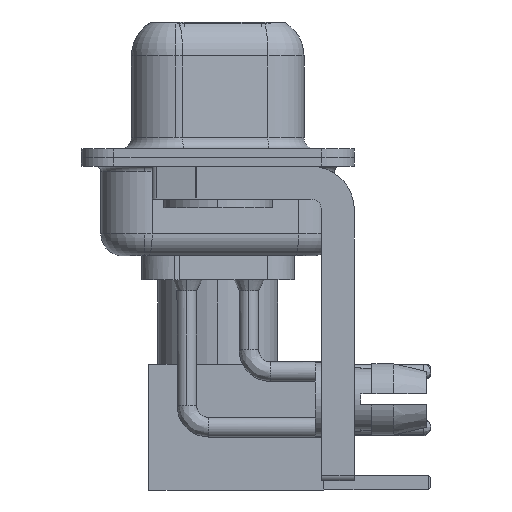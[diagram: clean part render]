
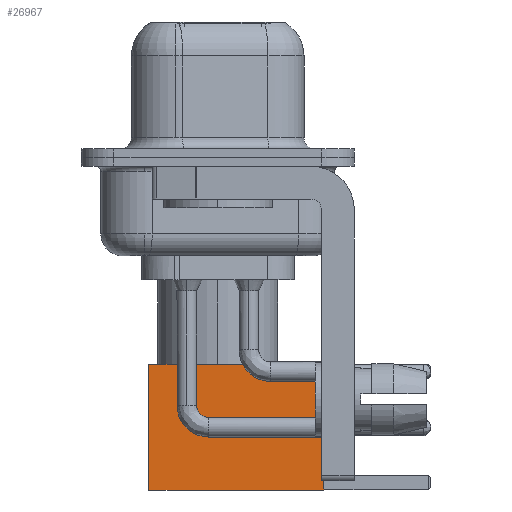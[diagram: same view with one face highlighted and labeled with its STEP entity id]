
A CAD part, left-side view. The second image highlights one B-rep face of the part: STEP entity #26967.
In plain terms, the highlighted face is planar.
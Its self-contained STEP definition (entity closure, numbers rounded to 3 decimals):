
#485 = CARTESIAN_POINT ( 'NONE',  ( 2.875, 2.875, 0. ) ) ;
#656 = VECTOR ( 'NONE', #3572, 1000. ) ;
#662 = LINE ( 'NONE', #13475, #1100 ) ;
#1100 = VECTOR ( 'NONE', #22975, 1000. ) ;
#1269 = CARTESIAN_POINT ( 'NONE',  ( -2.875, 2.875, 0. ) ) ;
#2920 = ORIENTED_EDGE ( 'NONE', *, *, #26882, .T. ) ;
#3572 = DIRECTION ( 'NONE',  ( 0., 0., -1. ) ) ;
#5492 = ORIENTED_EDGE ( 'NONE', *, *, #26355, .T. ) ;
#6103 = PLANE ( 'NONE',  #18853 ) ;
#7157 = VERTEX_POINT ( 'NONE', #485 ) ;
#7866 = CARTESIAN_POINT ( 'NONE',  ( 2.875, 2.875, 8. ) ) ;
#8279 = CARTESIAN_POINT ( 'NONE',  ( -2.875, 2.875, 0. ) ) ;
#9810 = LINE ( 'NONE', #1269, #19902 ) ;
#10529 = FACE_OUTER_BOUND ( 'NONE', #19339, .T. ) ;
#11374 = VERTEX_POINT ( 'NONE', #7866 ) ;
#12388 = DIRECTION ( 'NONE',  ( 0., 0., 1. ) ) ;
#12498 = ORIENTED_EDGE ( 'NONE', *, *, #13715, .F. ) ;
#12614 = VERTEX_POINT ( 'NONE', #14843 ) ;
#13475 = CARTESIAN_POINT ( 'NONE',  ( 0., 2.875, 0. ) ) ;
#13715 = EDGE_CURVE ( 'NONE', #12614, #16427, #9810, .T. ) ;
#14843 = CARTESIAN_POINT ( 'NONE',  ( -2.875, 2.875, 8. ) ) ;
#16333 = DIRECTION ( 'NONE',  ( -1., 0., 0. ) ) ;
#16427 = VERTEX_POINT ( 'NONE', #8279 ) ;
#16825 = CARTESIAN_POINT ( 'NONE',  ( 2.875, 2.875, 0. ) ) ;
#16898 = CARTESIAN_POINT ( 'NONE',  ( 0., 2.875, 8. ) ) ;
#18502 = DIRECTION ( 'NONE',  ( 0., 0., -1. ) ) ;
#18853 = AXIS2_PLACEMENT_3D ( 'NONE', #16825, #23356, #12388 ) ;
#19028 = LINE ( 'NONE', #16898, #24351 ) ;
#19339 = EDGE_LOOP ( 'NONE', ( #2920, #5492, #12498, #24939 ) ) ;
#19902 = VECTOR ( 'NONE', #18502, 1000. ) ;
#22975 = DIRECTION ( 'NONE',  ( -1., 0., 0. ) ) ;
#23356 = DIRECTION ( 'NONE',  ( 0., 1., 0. ) ) ;
#24351 = VECTOR ( 'NONE', #16333, 1000. ) ;
#24939 = ORIENTED_EDGE ( 'NONE', *, *, #27684, .F. ) ;
#25080 = LINE ( 'NONE', #25361, #656 ) ;
#25361 = CARTESIAN_POINT ( 'NONE',  ( 2.875, 2.875, 0. ) ) ;
#26355 = EDGE_CURVE ( 'NONE', #7157, #16427, #662, .T. ) ;
#26882 = EDGE_CURVE ( 'NONE', #11374, #7157, #25080, .T. ) ;
#26967 = ADVANCED_FACE ( 'NONE', ( #10529 ), #6103, .T. ) ;
#27684 = EDGE_CURVE ( 'NONE', #11374, #12614, #19028, .T. ) ;
